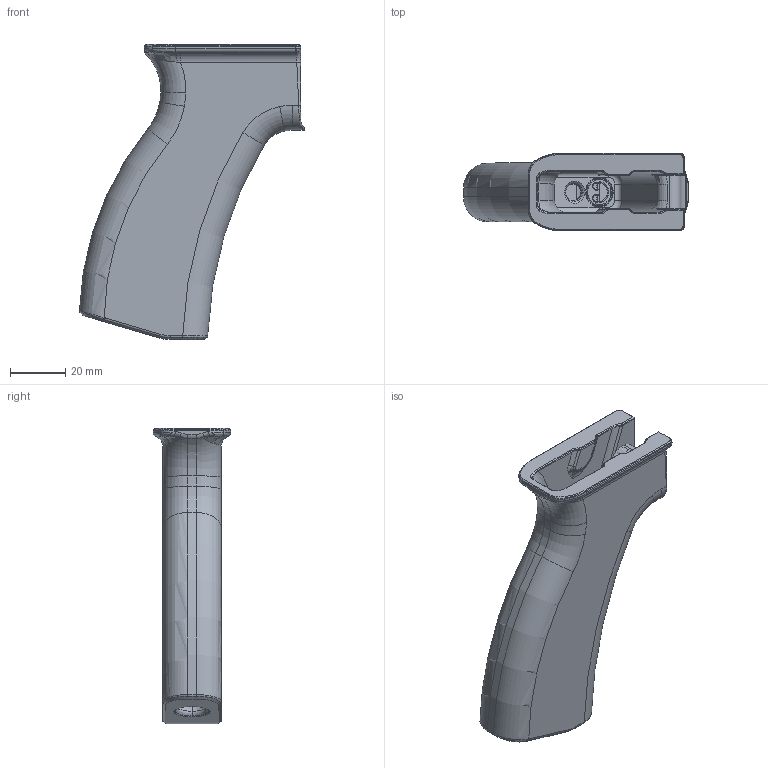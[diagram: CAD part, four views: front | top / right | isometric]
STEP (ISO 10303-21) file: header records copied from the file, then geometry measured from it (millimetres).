
FILE_DESCRIPTION(/* description */ (''),/* implementation_level */ '2;1');
FILE_NAME(/* name */ 'Standard.step',/* time_stamp */ '2021-09-20T01:27:09-04:00',/* author */ (''),/* organization */ (''),/* preprocessor_version */ 'ST-DEVELOPER v18.1',/* originating_system */ 'Autodesk Translation Framework v10.10.0.1391',/* authorisation */ '');
FILE_SCHEMA (('AUTOMOTIVE_DESIGN { 1 0 10303 214 3 1 1 }'));
Length unit declared in the file: millimetre
Products named in the file (1): Standard
Bounding box: 81.2 x 28 x 106.49 mm (x, y, z)
Volume: 52830.8 mm3; surface area: 25505.7 mm2
Topology: 1 solids, 1 shells, 458 faces, 1102 edges, 642 vertices
Faces by surface type: bspline 240, cylinder 103, torus 57, plane 52, cone 6
Entity records: 18684 total; most frequent: CARTESIAN_POINT 9423, ORIENTED_EDGE 2180, DIRECTION 1487, EDGE_CURVE 1090, VERTEX_POINT 642, AXIS2_PLACEMENT_3D 611, EDGE_LOOP 468, FACE_OUTER_BOUND 458
